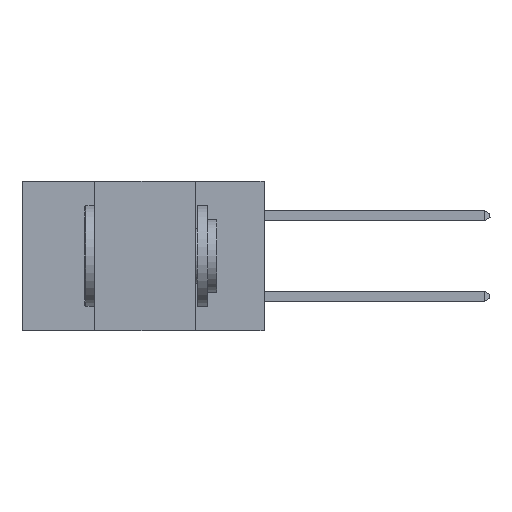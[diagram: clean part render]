
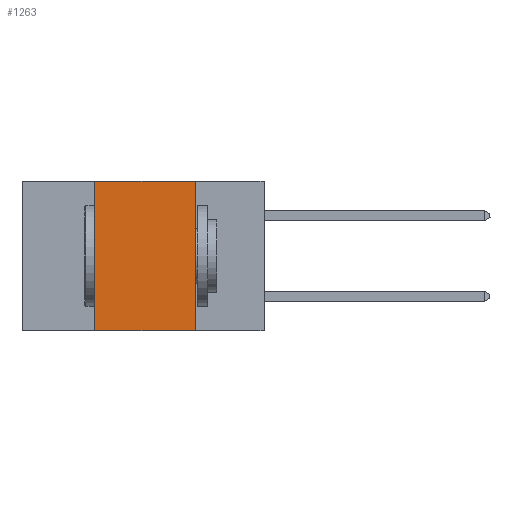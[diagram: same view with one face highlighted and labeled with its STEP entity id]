
A CAD part, left-side view. The second image highlights one B-rep face of the part: STEP entity #1263.
In plain terms, the highlighted planar face has unit normal (-1, 0, 0).
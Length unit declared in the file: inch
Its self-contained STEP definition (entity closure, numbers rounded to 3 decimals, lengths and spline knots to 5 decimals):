
#352 = ORIENTED_EDGE ( 'NONE', *, *, #2014, .F. ) ;
#818 = CARTESIAN_POINT ( 'NONE',  ( 0., 0.17, 0. ) ) ;
#1248 = EDGE_CURVE ( 'NONE', #3580, #2960, #6997, .T. ) ;
#1263 = ADVANCED_FACE ( 'NONE', ( #9008 ), #1632, .F. ) ;
#1632 = PLANE ( 'NONE',  #7004 ) ;
#2014 = EDGE_CURVE ( 'NONE', #15514, #6960, #8777, .T. ) ;
#2904 = DIRECTION ( 'NONE',  ( 1., 0., 0. ) ) ;
#2960 = VERTEX_POINT ( 'NONE', #8020 ) ;
#3010 = CARTESIAN_POINT ( 'NONE',  ( 0., 0.6, -0.37 ) ) ;
#3580 = VERTEX_POINT ( 'NONE', #4849 ) ;
#3589 = VECTOR ( 'NONE', #12004, 39.37008 ) ;
#3903 = LINE ( 'NONE', #9793, #8124 ) ;
#4849 = CARTESIAN_POINT ( 'NONE',  ( 0., 0.42, -0.37 ) ) ;
#4860 = VECTOR ( 'NONE', #10992, 39.37008 ) ;
#5248 = ORIENTED_EDGE ( 'NONE', *, *, #12737, .F. ) ;
#5524 = EDGE_CURVE ( 'NONE', #3580, #15514, #3903, .T. ) ;
#6509 = CARTESIAN_POINT ( 'NONE',  ( 0., 0.6, 0. ) ) ;
#6960 = VERTEX_POINT ( 'NONE', #10514 ) ;
#6997 = LINE ( 'NONE', #3010, #3589 ) ;
#7004 = AXIS2_PLACEMENT_3D ( 'NONE', #10562, #2904, #13123 ) ;
#8020 = CARTESIAN_POINT ( 'NONE',  ( 0., 0.17, -0.37 ) ) ;
#8124 = VECTOR ( 'NONE', #11082, 39.37008 ) ;
#8777 = LINE ( 'NONE', #6509, #13536 ) ;
#9008 = FACE_OUTER_BOUND ( 'NONE', #16396, .T. ) ;
#9145 = DIRECTION ( 'NONE',  ( 0., -1., 0. ) ) ;
#9668 = LINE ( 'NONE', #818, #4860 ) ;
#9793 = CARTESIAN_POINT ( 'NONE',  ( 0., 0.42, 0. ) ) ;
#10514 = CARTESIAN_POINT ( 'NONE',  ( 0., 0.17, 0. ) ) ;
#10562 = CARTESIAN_POINT ( 'NONE',  ( 0., 0.6, 0. ) ) ;
#10942 = ORIENTED_EDGE ( 'NONE', *, *, #1248, .T. ) ;
#10992 = DIRECTION ( 'NONE',  ( 0., 0., -1. ) ) ;
#11082 = DIRECTION ( 'NONE',  ( 0., 0., 1. ) ) ;
#12004 = DIRECTION ( 'NONE',  ( 0., -1., 0. ) ) ;
#12737 = EDGE_CURVE ( 'NONE', #6960, #2960, #9668, .T. ) ;
#13123 = DIRECTION ( 'NONE',  ( 0., 0., -1. ) ) ;
#13536 = VECTOR ( 'NONE', #9145, 39.37008 ) ;
#15013 = CARTESIAN_POINT ( 'NONE',  ( 0., 0.42, 0. ) ) ;
#15514 = VERTEX_POINT ( 'NONE', #15013 ) ;
#15749 = ORIENTED_EDGE ( 'NONE', *, *, #5524, .F. ) ;
#16396 = EDGE_LOOP ( 'NONE', ( #5248, #352, #15749, #10942 ) ) ;
